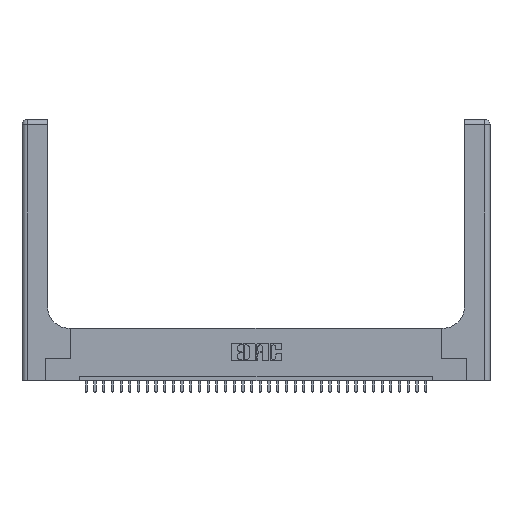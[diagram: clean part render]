
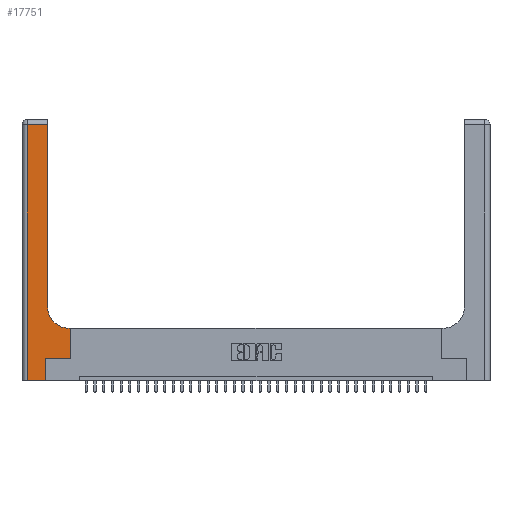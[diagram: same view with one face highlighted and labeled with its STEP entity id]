
A CAD part, top view. The second image highlights one B-rep face of the part: STEP entity #17751.
In plain terms, the highlighted planar face has unit normal (0, 0, 1).
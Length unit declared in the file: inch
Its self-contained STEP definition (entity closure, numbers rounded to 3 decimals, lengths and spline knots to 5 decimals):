
#235 = LINE ( 'NONE', #33418, #6677 ) ;
#588 = EDGE_CURVE ( 'NONE', #12627, #25737, #12127, .T. ) ;
#1763 = DIRECTION ( 'NONE',  ( 1., 0., 0. ) ) ;
#1775 = CARTESIAN_POINT ( 'NONE',  ( 0.5585, 0.6, 0.37 ) ) ;
#1826 = CARTESIAN_POINT ( 'NONE',  ( 0.5415, 0.6, 0.37 ) ) ;
#2004 = PLANE ( 'NONE',  #13416 ) ;
#2856 = EDGE_CURVE ( 'NONE', #5806, #13326, #31731, .T. ) ;
#3104 = CARTESIAN_POINT ( 'NONE',  ( 0.06, 0., 0.37 ) ) ;
#3509 = CARTESIAN_POINT ( 'NONE',  ( 0.2915, 0.6, 0.37 ) ) ;
#3599 = LINE ( 'NONE', #6096, #32847 ) ;
#3966 = VECTOR ( 'NONE', #33583, 39.37008 ) ;
#4136 = ORIENTED_EDGE ( 'NONE', *, *, #5443, .T. ) ;
#4218 = EDGE_LOOP ( 'NONE', ( #4136, #30232, #24328, #13189, #6288, #13367, #33558, #33536, #27707 ) ) ;
#4572 = CARTESIAN_POINT ( 'NONE',  ( 0.5415, 0.85, 0.37 ) ) ;
#4742 = LINE ( 'NONE', #30901, #18514 ) ;
#5443 = EDGE_CURVE ( 'NONE', #26322, #23549, #12806, .T. ) ;
#5806 = VERTEX_POINT ( 'NONE', #1775 ) ;
#6096 = CARTESIAN_POINT ( 'NONE',  ( 0.269, 0., 0.37 ) ) ;
#6251 = AXIS2_PLACEMENT_3D ( 'NONE', #4572, #34739, #18273 ) ;
#6288 = ORIENTED_EDGE ( 'NONE', *, *, #14778, .T. ) ;
#6557 = CARTESIAN_POINT ( 'NONE',  ( 0., 0., 0.37 ) ) ;
#6677 = VECTOR ( 'NONE', #25386, 39.37008 ) ;
#7988 = VERTEX_POINT ( 'NONE', #24126 ) ;
#10252 = CARTESIAN_POINT ( 'NONE',  ( 0.2915, 0.85, 0.37 ) ) ;
#12127 = LINE ( 'NONE', #15174, #3966 ) ;
#12364 = CARTESIAN_POINT ( 'NONE',  ( 0., 3., 0.37 ) ) ;
#12627 = VERTEX_POINT ( 'NONE', #21305 ) ;
#12704 = DIRECTION ( 'NONE',  ( -1., 0., 0. ) ) ;
#12806 = LINE ( 'NONE', #32196, #30394 ) ;
#13008 = CARTESIAN_POINT ( 'NONE',  ( 0.269, 0.25, 0.37 ) ) ;
#13189 = ORIENTED_EDGE ( 'NONE', *, *, #28406, .T. ) ;
#13326 = VERTEX_POINT ( 'NONE', #1826 ) ;
#13367 = ORIENTED_EDGE ( 'NONE', *, *, #26561, .T. ) ;
#13416 = AXIS2_PLACEMENT_3D ( 'NONE', #12364, #26079, #28580 ) ;
#13556 = FACE_OUTER_BOUND ( 'NONE', #4218, .T. ) ;
#14778 = EDGE_CURVE ( 'NONE', #7988, #20350, #3599, .T. ) ;
#15174 = CARTESIAN_POINT ( 'NONE',  ( 0.06, 3., 0.37 ) ) ;
#15444 = CARTESIAN_POINT ( 'NONE',  ( 0.5585, 0.25, 0.37 ) ) ;
#15451 = VECTOR ( 'NONE', #28378, 39.37008 ) ;
#17429 = DIRECTION ( 'NONE',  ( 0., 1., 0. ) ) ;
#17751 = ADVANCED_FACE ( 'NONE', ( #13556 ), #2004, .F. ) ;
#17830 = DIRECTION ( 'NONE',  ( 0., 1., 0. ) ) ;
#18273 = DIRECTION ( 'NONE',  ( 1., 0., 0. ) ) ;
#18486 = DIRECTION ( 'NONE',  ( 0., 1., 0. ) ) ;
#18514 = VECTOR ( 'NONE', #17830, 39.37008 ) ;
#20327 = EDGE_CURVE ( 'NONE', #26351, #5806, #4742, .T. ) ;
#20350 = VERTEX_POINT ( 'NONE', #13008 ) ;
#21034 = CIRCLE ( 'NONE', #6251, 0.25 ) ;
#21181 = EDGE_CURVE ( 'NONE', #23549, #12627, #29693, .T. ) ;
#21305 = CARTESIAN_POINT ( 'NONE',  ( 0.06, 2.94, 0.37 ) ) ;
#21840 = EDGE_CURVE ( 'NONE', #13326, #26322, #21034, .T. ) ;
#23549 = VERTEX_POINT ( 'NONE', #26360 ) ;
#24126 = CARTESIAN_POINT ( 'NONE',  ( 0.269, 0., 0.37 ) ) ;
#24328 = ORIENTED_EDGE ( 'NONE', *, *, #588, .T. ) ;
#24563 = VECTOR ( 'NONE', #1763, 39.37008 ) ;
#25386 = DIRECTION ( 'NONE',  ( 1., 0., 0. ) ) ;
#25737 = VERTEX_POINT ( 'NONE', #3104 ) ;
#26079 = DIRECTION ( 'NONE',  ( 0., 0., -1. ) ) ;
#26261 = VECTOR ( 'NONE', #12704, 39.37008 ) ;
#26322 = VERTEX_POINT ( 'NONE', #10252 ) ;
#26351 = VERTEX_POINT ( 'NONE', #15444 ) ;
#26360 = CARTESIAN_POINT ( 'NONE',  ( 0.2915, 2.94, 0.37 ) ) ;
#26561 = EDGE_CURVE ( 'NONE', #20350, #26351, #235, .T. ) ;
#27707 = ORIENTED_EDGE ( 'NONE', *, *, #21840, .T. ) ;
#28378 = DIRECTION ( 'NONE',  ( -1., 0., 0. ) ) ;
#28406 = EDGE_CURVE ( 'NONE', #25737, #7988, #28876, .T. ) ;
#28580 = DIRECTION ( 'NONE',  ( -1., 0., 0. ) ) ;
#28876 = LINE ( 'NONE', #6557, #24563 ) ;
#29693 = LINE ( 'NONE', #34447, #26261 ) ;
#30232 = ORIENTED_EDGE ( 'NONE', *, *, #21181, .T. ) ;
#30394 = VECTOR ( 'NONE', #18486, 39.37008 ) ;
#30901 = CARTESIAN_POINT ( 'NONE',  ( 0.5585, 0.25, 0.37 ) ) ;
#31731 = LINE ( 'NONE', #3509, #15451 ) ;
#32196 = CARTESIAN_POINT ( 'NONE',  ( 0.2915, 3., 0.37 ) ) ;
#32847 = VECTOR ( 'NONE', #17429, 39.37008 ) ;
#33418 = CARTESIAN_POINT ( 'NONE',  ( 0.269, 0.25, 0.37 ) ) ;
#33536 = ORIENTED_EDGE ( 'NONE', *, *, #2856, .T. ) ;
#33558 = ORIENTED_EDGE ( 'NONE', *, *, #20327, .T. ) ;
#33583 = DIRECTION ( 'NONE',  ( 0., -1., 0. ) ) ;
#34447 = CARTESIAN_POINT ( 'NONE',  ( 0., 2.94, 0.37 ) ) ;
#34739 = DIRECTION ( 'NONE',  ( 0., 0., -1. ) ) ;
